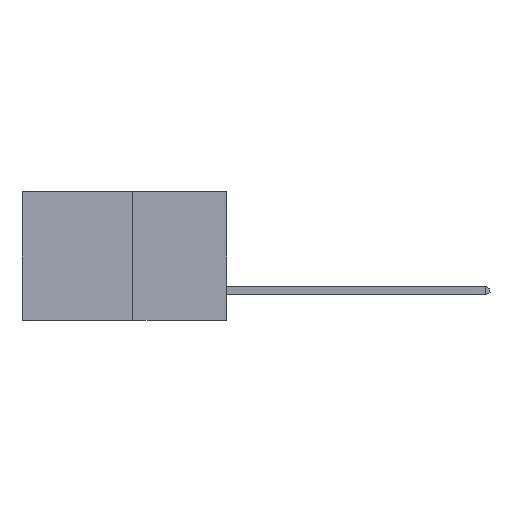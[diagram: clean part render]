
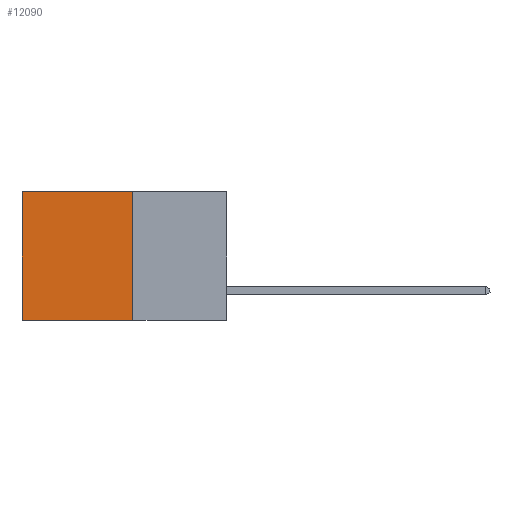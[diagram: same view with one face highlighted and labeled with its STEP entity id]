
A CAD part, left-side view. The second image highlights one B-rep face of the part: STEP entity #12090.
In plain terms, the highlighted planar face has unit normal (-1, 0, 0).
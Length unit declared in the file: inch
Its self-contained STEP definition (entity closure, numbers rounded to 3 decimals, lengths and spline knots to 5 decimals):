
#130 = VERTEX_POINT ( 'NONE', #1961 ) ;
#173 = VERTEX_POINT ( 'NONE', #6791 ) ;
#423 = CARTESIAN_POINT ( 'NONE',  ( 0.277, 0.59, -0.37 ) ) ;
#913 = VERTEX_POINT ( 'NONE', #423 ) ;
#1961 = CARTESIAN_POINT ( 'NONE',  ( 0.277, 0.27, 0. ) ) ;
#2512 = PLANE ( 'NONE',  #6475 ) ;
#2588 = VECTOR ( 'NONE', #7839, 39.37008 ) ;
#2594 = CARTESIAN_POINT ( 'NONE',  ( 0.277, 0.59, -0.37 ) ) ;
#2612 = CARTESIAN_POINT ( 'NONE',  ( 0.277, 0.27, -0.37 ) ) ;
#3557 = DIRECTION ( 'NONE',  ( 0., 0., -1. ) ) ;
#3653 = DIRECTION ( 'NONE',  ( 0., 0., -1. ) ) ;
#3921 = LINE ( 'NONE', #6574, #9129 ) ;
#5364 = LINE ( 'NONE', #2594, #2588 ) ;
#6002 = LINE ( 'NONE', #2612, #8469 ) ;
#6229 = FACE_OUTER_BOUND ( 'NONE', #12237, .T. ) ;
#6385 = DIRECTION ( 'NONE',  ( 0., 1., 0. ) ) ;
#6475 = AXIS2_PLACEMENT_3D ( 'NONE', #11720, #9754, #3557 ) ;
#6574 = CARTESIAN_POINT ( 'NONE',  ( 0.277, 0.27, -0.37 ) ) ;
#6791 = CARTESIAN_POINT ( 'NONE',  ( 0.277, 0.59, 0. ) ) ;
#7245 = ORIENTED_EDGE ( 'NONE', *, *, #7960, .T. ) ;
#7256 = CARTESIAN_POINT ( 'NONE',  ( 0.277, 0.27, -0.37 ) ) ;
#7258 = EDGE_CURVE ( 'NONE', #130, #7558, #6002, .T. ) ;
#7558 = VERTEX_POINT ( 'NONE', #7256 ) ;
#7839 = DIRECTION ( 'NONE',  ( 0., 0., -1. ) ) ;
#7960 = EDGE_CURVE ( 'NONE', #173, #913, #5364, .T. ) ;
#8469 = VECTOR ( 'NONE', #3653, 39.37008 ) ;
#9005 = EDGE_CURVE ( 'NONE', #130, #173, #10609, .T. ) ;
#9129 = VECTOR ( 'NONE', #11642, 39.37008 ) ;
#9754 = DIRECTION ( 'NONE',  ( 1., 0., 0. ) ) ;
#9945 = ORIENTED_EDGE ( 'NONE', *, *, #13100, .F. ) ;
#10609 = LINE ( 'NONE', #13433, #13247 ) ;
#11642 = DIRECTION ( 'NONE',  ( 0., 1., 0. ) ) ;
#11720 = CARTESIAN_POINT ( 'NONE',  ( 0.277, 0.27, -0.37 ) ) ;
#12090 = ADVANCED_FACE ( 'NONE', ( #6229 ), #2512, .F. ) ;
#12237 = EDGE_LOOP ( 'NONE', ( #7245, #9945, #12598, #12897 ) ) ;
#12598 = ORIENTED_EDGE ( 'NONE', *, *, #7258, .F. ) ;
#12897 = ORIENTED_EDGE ( 'NONE', *, *, #9005, .T. ) ;
#13100 = EDGE_CURVE ( 'NONE', #7558, #913, #3921, .T. ) ;
#13247 = VECTOR ( 'NONE', #6385, 39.37008 ) ;
#13433 = CARTESIAN_POINT ( 'NONE',  ( 0.277, 0.27, 0. ) ) ;
